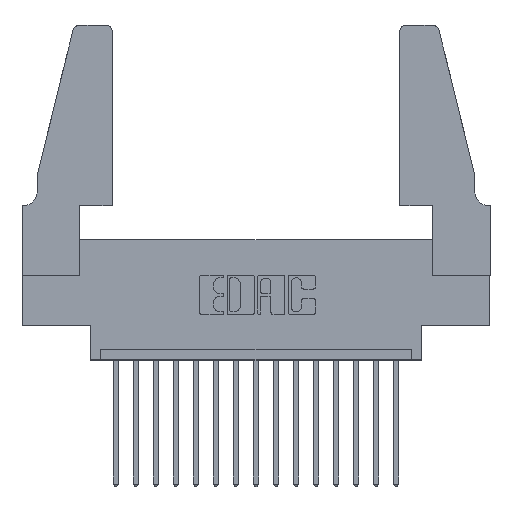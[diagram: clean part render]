
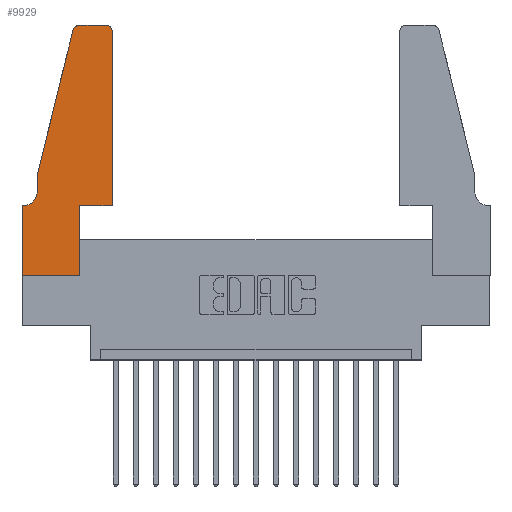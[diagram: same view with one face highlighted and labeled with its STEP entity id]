
A CAD part, top view. The second image highlights one B-rep face of the part: STEP entity #9929.
In plain terms, the highlighted planar face has unit normal (0, 0, 1).
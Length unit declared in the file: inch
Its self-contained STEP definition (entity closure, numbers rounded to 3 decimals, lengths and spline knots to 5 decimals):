
#32 = EDGE_CURVE ( 'NONE', #13220, #7005, #16553, .T. ) ;
#64 = FACE_OUTER_BOUND ( 'NONE', #7839, .T. ) ;
#151 = CARTESIAN_POINT ( 'NONE',  ( 0.4205, 1.22, 0.37 ) ) ;
#251 = ORIENTED_EDGE ( 'NONE', *, *, #665, .T. ) ;
#402 = VERTEX_POINT ( 'NONE', #15556 ) ;
#607 = VERTEX_POINT ( 'NONE', #9205 ) ;
#665 = EDGE_CURVE ( 'NONE', #7005, #3629, #2069, .T. ) ;
#794 = ORIENTED_EDGE ( 'NONE', *, *, #2736, .T. ) ;
#983 = AXIS2_PLACEMENT_3D ( 'NONE', #8108, #13229, #10550 ) ;
#1021 = DIRECTION ( 'NONE',  ( 0., 0., -1. ) ) ;
#1433 = VECTOR ( 'NONE', #12083, 39.37008 ) ;
#1529 = VERTEX_POINT ( 'NONE', #15147 ) ;
#1758 = DIRECTION ( 'NONE',  ( 0., -1., 0. ) ) ;
#1796 = ORIENTED_EDGE ( 'NONE', *, *, #4786, .T. ) ;
#2069 = LINE ( 'NONE', #2610, #9350 ) ;
#2233 = ORIENTED_EDGE ( 'NONE', *, *, #10554, .T. ) ;
#2477 = VECTOR ( 'NONE', #4924, 39.37008 ) ;
#2610 = CARTESIAN_POINT ( 'NONE',  ( 0.2605, 1.25, 0.37 ) ) ;
#2719 = ORIENTED_EDGE ( 'NONE', *, *, #6911, .T. ) ;
#2736 = EDGE_CURVE ( 'NONE', #10651, #13220, #4522, .T. ) ;
#3005 = CARTESIAN_POINT ( 'NONE',  ( 0.4505, 1.22, 0.37 ) ) ;
#3309 = CARTESIAN_POINT ( 'NONE',  ( 0.0755, 0.42, 0.37 ) ) ;
#3422 = DIRECTION ( 'NONE',  ( -0.239, -0.971, 0. ) ) ;
#3533 = ORIENTED_EDGE ( 'NONE', *, *, #11899, .T. ) ;
#3629 = VERTEX_POINT ( 'NONE', #3967 ) ;
#3937 = PLANE ( 'NONE',  #983 ) ;
#3967 = CARTESIAN_POINT ( 'NONE',  ( 0.284, 1.25, 0.37 ) ) ;
#4106 = VERTEX_POINT ( 'NONE', #16531 ) ;
#4161 = LINE ( 'NONE', #15111, #7926 ) ;
#4416 = CARTESIAN_POINT ( 'NONE',  ( 0.4505, 0.35, 0.37 ) ) ;
#4522 = LINE ( 'NONE', #4416, #17028 ) ;
#4695 = LINE ( 'NONE', #5911, #13223 ) ;
#4786 = EDGE_CURVE ( 'NONE', #8351, #10423, #11286, .T. ) ;
#4816 = LINE ( 'NONE', #13809, #9993 ) ;
#4924 = DIRECTION ( 'NONE',  ( -1., 0., 0. ) ) ;
#4965 = CARTESIAN_POINT ( 'NONE',  ( 0.0055, 0.42, 0.37 ) ) ;
#5128 = CARTESIAN_POINT ( 'NONE',  ( 0.4505, 0.35, 0.37 ) ) ;
#5911 = CARTESIAN_POINT ( 'NONE',  ( 0.0755, 0.5, 0.37 ) ) ;
#5943 = ORIENTED_EDGE ( 'NONE', *, *, #15117, .T. ) ;
#6148 = CARTESIAN_POINT ( 'NONE',  ( 0.284, 1.22, 0.37 ) ) ;
#6230 = EDGE_CURVE ( 'NONE', #3629, #607, #13938, .T. ) ;
#6877 = VECTOR ( 'NONE', #1758, 39.37008 ) ;
#6911 = EDGE_CURVE ( 'NONE', #402, #7001, #10361, .T. ) ;
#7001 = VERTEX_POINT ( 'NONE', #13055 ) ;
#7005 = VERTEX_POINT ( 'NONE', #15861 ) ;
#7839 = EDGE_LOOP ( 'NONE', ( #251, #17007, #3533, #13976, #1796, #10906, #15145, #2719, #2233, #5943, #794, #15626 ) ) ;
#7926 = VECTOR ( 'NONE', #3422, 39.37008 ) ;
#7931 = LINE ( 'NONE', #13550, #6877 ) ;
#8108 = CARTESIAN_POINT ( 'NONE',  ( 0., 0.35, 0.37 ) ) ;
#8264 = LINE ( 'NONE', #14677, #2477 ) ;
#8351 = VERTEX_POINT ( 'NONE', #3309 ) ;
#8552 = DIRECTION ( 'NONE',  ( 0., -1., 0. ) ) ;
#8796 = DIRECTION ( 'NONE',  ( 0., 0., 1. ) ) ;
#9205 = CARTESIAN_POINT ( 'NONE',  ( 0.25487, 1.22718, 0.37 ) ) ;
#9350 = VECTOR ( 'NONE', #14628, 39.37008 ) ;
#9435 = DIRECTION ( 'NONE',  ( 0., 0., 1. ) ) ;
#9920 = VECTOR ( 'NONE', #10083, 39.37008 ) ;
#9929 = ADVANCED_FACE ( 'NONE', ( #64 ), #3937, .T. ) ;
#9993 = VECTOR ( 'NONE', #15153, 39.37008 ) ;
#10083 = DIRECTION ( 'NONE',  ( 1., 0., 0. ) ) ;
#10361 = LINE ( 'NONE', #11483, #9920 ) ;
#10423 = VERTEX_POINT ( 'NONE', #11785 ) ;
#10550 = DIRECTION ( 'NONE',  ( 1., 0., 0. ) ) ;
#10554 = EDGE_CURVE ( 'NONE', #7001, #1529, #4816, .T. ) ;
#10651 = VERTEX_POINT ( 'NONE', #5128 ) ;
#10710 = CARTESIAN_POINT ( 'NONE',  ( 0.4505, 0.35, 0.37 ) ) ;
#10906 = ORIENTED_EDGE ( 'NONE', *, *, #14794, .T. ) ;
#11213 = AXIS2_PLACEMENT_3D ( 'NONE', #4965, #1021, #14071 ) ;
#11286 = CIRCLE ( 'NONE', #11213, 0.07 ) ;
#11369 = LINE ( 'NONE', #10710, #1433 ) ;
#11483 = CARTESIAN_POINT ( 'NONE',  ( 0., 0., 0.37 ) ) ;
#11785 = CARTESIAN_POINT ( 'NONE',  ( 0.0055, 0.35, 0.37 ) ) ;
#11899 = EDGE_CURVE ( 'NONE', #607, #15633, #4161, .T. ) ;
#12083 = DIRECTION ( 'NONE',  ( 1., 0., 0. ) ) ;
#12193 = DIRECTION ( 'NONE',  ( 1., 0., 0. ) ) ;
#13055 = CARTESIAN_POINT ( 'NONE',  ( 0.2865, 0., 0.37 ) ) ;
#13220 = VERTEX_POINT ( 'NONE', #3005 ) ;
#13223 = VECTOR ( 'NONE', #8552, 39.37008 ) ;
#13229 = DIRECTION ( 'NONE',  ( 0., 0., 1. ) ) ;
#13550 = CARTESIAN_POINT ( 'NONE',  ( 0., 0., 0.37 ) ) ;
#13592 = EDGE_CURVE ( 'NONE', #4106, #402, #7931, .T. ) ;
#13809 = CARTESIAN_POINT ( 'NONE',  ( 0.2865, 0.35, 0.37 ) ) ;
#13938 = CIRCLE ( 'NONE', #15346, 0.03 ) ;
#13944 = DIRECTION ( 'NONE',  ( 0., 1., 0. ) ) ;
#13976 = ORIENTED_EDGE ( 'NONE', *, *, #16239, .T. ) ;
#14071 = DIRECTION ( 'NONE',  ( -1., 0., 0. ) ) ;
#14260 = CARTESIAN_POINT ( 'NONE',  ( 0.0755, 0.5, 0.37 ) ) ;
#14628 = DIRECTION ( 'NONE',  ( -1., 0., 0. ) ) ;
#14677 = CARTESIAN_POINT ( 'NONE',  ( 0.0755, 0.35, 0.37 ) ) ;
#14794 = EDGE_CURVE ( 'NONE', #10423, #4106, #8264, .T. ) ;
#15111 = CARTESIAN_POINT ( 'NONE',  ( 0.0755, 0.5, 0.37 ) ) ;
#15117 = EDGE_CURVE ( 'NONE', #1529, #10651, #11369, .T. ) ;
#15145 = ORIENTED_EDGE ( 'NONE', *, *, #13592, .T. ) ;
#15147 = CARTESIAN_POINT ( 'NONE',  ( 0.2865, 0.35, 0.37 ) ) ;
#15153 = DIRECTION ( 'NONE',  ( 0., 1., 0. ) ) ;
#15346 = AXIS2_PLACEMENT_3D ( 'NONE', #6148, #8796, #16602 ) ;
#15556 = CARTESIAN_POINT ( 'NONE',  ( 0., 0., 0.37 ) ) ;
#15626 = ORIENTED_EDGE ( 'NONE', *, *, #32, .T. ) ;
#15633 = VERTEX_POINT ( 'NONE', #14260 ) ;
#15861 = CARTESIAN_POINT ( 'NONE',  ( 0.4205, 1.25, 0.37 ) ) ;
#16239 = EDGE_CURVE ( 'NONE', #15633, #8351, #4695, .T. ) ;
#16531 = CARTESIAN_POINT ( 'NONE',  ( 0., 0.35, 0.37 ) ) ;
#16553 = CIRCLE ( 'NONE', #16633, 0.03 ) ;
#16602 = DIRECTION ( 'NONE',  ( 1., 0., 0. ) ) ;
#16633 = AXIS2_PLACEMENT_3D ( 'NONE', #151, #9435, #12193 ) ;
#17007 = ORIENTED_EDGE ( 'NONE', *, *, #6230, .T. ) ;
#17028 = VECTOR ( 'NONE', #13944, 39.37008 ) ;
